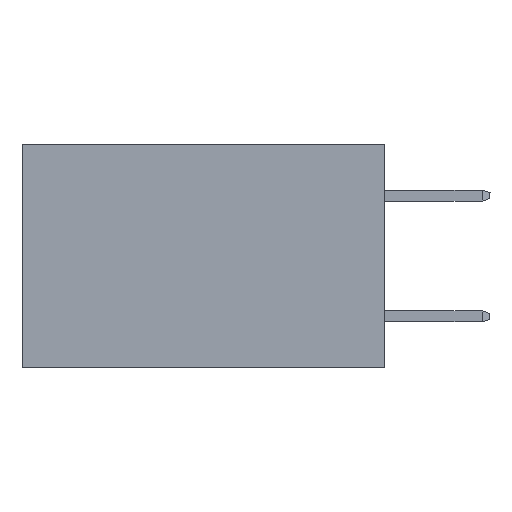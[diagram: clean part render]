
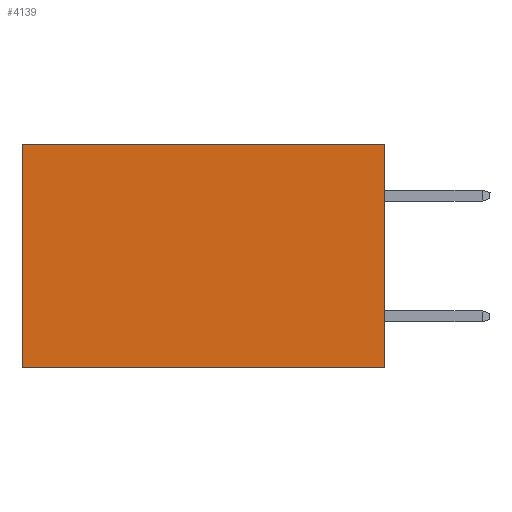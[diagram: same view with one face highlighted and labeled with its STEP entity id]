
A CAD part, left-side view. The second image highlights one B-rep face of the part: STEP entity #4139.
In plain terms, the highlighted planar face has unit normal (-1, 0, 0).
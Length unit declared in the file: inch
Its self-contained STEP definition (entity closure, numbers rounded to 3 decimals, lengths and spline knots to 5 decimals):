
#966 = EDGE_CURVE ( 'NONE', #12926, #8299, #6212, .T. ) ;
#1250 = CARTESIAN_POINT ( 'NONE',  ( 0.298, 0., 0. ) ) ;
#1905 = CARTESIAN_POINT ( 'NONE',  ( 0.298, 0., 0. ) ) ;
#2008 = ORIENTED_EDGE ( 'NONE', *, *, #9113, .T. ) ;
#2447 = LINE ( 'NONE', #1905, #10688 ) ;
#3022 = CARTESIAN_POINT ( 'NONE',  ( 0.298, 0.6, 0. ) ) ;
#3100 = DIRECTION ( 'NONE',  ( 0., 1., 0. ) ) ;
#3454 = VERTEX_POINT ( 'NONE', #8632 ) ;
#4139 = ADVANCED_FACE ( 'NONE', ( #11578 ), #13174, .F. ) ;
#4283 = CARTESIAN_POINT ( 'NONE',  ( 0.298, 0., -0.37 ) ) ;
#4290 = EDGE_CURVE ( 'NONE', #8481, #12926, #8945, .T. ) ;
#5021 = CARTESIAN_POINT ( 'NONE',  ( 0.298, 0., -0.37 ) ) ;
#5107 = CARTESIAN_POINT ( 'NONE',  ( 0.298, 0., 0. ) ) ;
#6212 = LINE ( 'NONE', #5021, #11145 ) ;
#6512 = ORIENTED_EDGE ( 'NONE', *, *, #4290, .F. ) ;
#6877 = CARTESIAN_POINT ( 'NONE',  ( 0.298, 0., 0. ) ) ;
#7262 = DIRECTION ( 'NONE',  ( 0., 1., 0. ) ) ;
#7913 = EDGE_LOOP ( 'NONE', ( #2008, #10735, #6512, #8286 ) ) ;
#8111 = DIRECTION ( 'NONE',  ( 0., 0., -1. ) ) ;
#8286 = ORIENTED_EDGE ( 'NONE', *, *, #10731, .T. ) ;
#8299 = VERTEX_POINT ( 'NONE', #10266 ) ;
#8481 = VERTEX_POINT ( 'NONE', #1250 ) ;
#8632 = CARTESIAN_POINT ( 'NONE',  ( 0.298, 0.6, 0. ) ) ;
#8945 = LINE ( 'NONE', #5107, #9630 ) ;
#9084 = DIRECTION ( 'NONE',  ( 1., 0., 0. ) ) ;
#9113 = EDGE_CURVE ( 'NONE', #3454, #8299, #12533, .T. ) ;
#9630 = VECTOR ( 'NONE', #8111, 39.37008 ) ;
#10155 = DIRECTION ( 'NONE',  ( 0., 0., -1. ) ) ;
#10266 = CARTESIAN_POINT ( 'NONE',  ( 0.298, 0.6, -0.37 ) ) ;
#10362 = DIRECTION ( 'NONE',  ( 0., 0., -1. ) ) ;
#10688 = VECTOR ( 'NONE', #3100, 39.37008 ) ;
#10731 = EDGE_CURVE ( 'NONE', #8481, #3454, #2447, .T. ) ;
#10735 = ORIENTED_EDGE ( 'NONE', *, *, #966, .F. ) ;
#11012 = AXIS2_PLACEMENT_3D ( 'NONE', #6877, #9084, #10155 ) ;
#11049 = VECTOR ( 'NONE', #10362, 39.37008 ) ;
#11145 = VECTOR ( 'NONE', #7262, 39.37008 ) ;
#11578 = FACE_OUTER_BOUND ( 'NONE', #7913, .T. ) ;
#12533 = LINE ( 'NONE', #3022, #11049 ) ;
#12926 = VERTEX_POINT ( 'NONE', #4283 ) ;
#13174 = PLANE ( 'NONE',  #11012 ) ;
